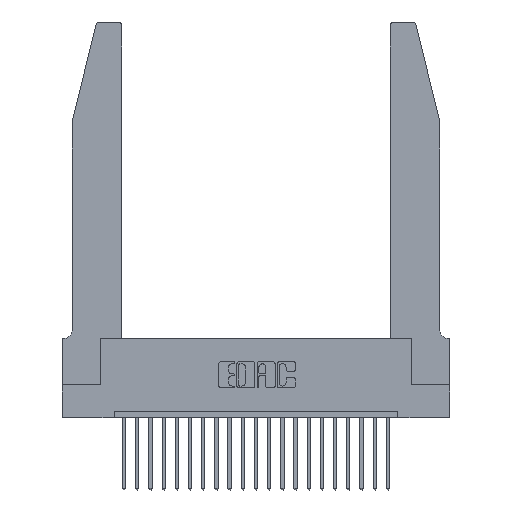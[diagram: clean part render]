
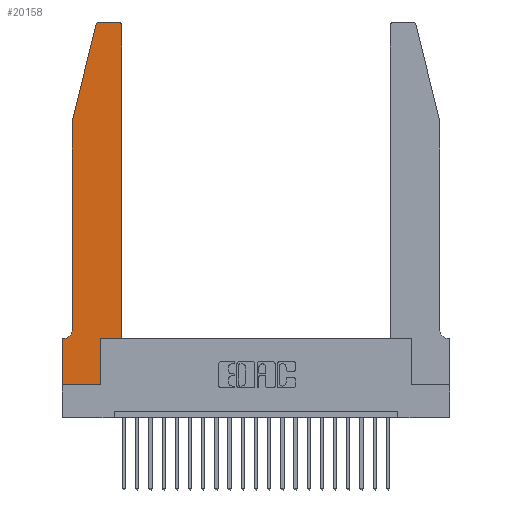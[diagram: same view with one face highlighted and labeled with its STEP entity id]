
A CAD part, top view. The second image highlights one B-rep face of the part: STEP entity #20158.
In plain terms, the highlighted planar face has unit normal (0, 0, 1).
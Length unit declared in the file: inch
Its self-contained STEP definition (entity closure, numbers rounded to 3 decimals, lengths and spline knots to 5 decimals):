
#213 = VECTOR ( 'NONE', #15141, 39.37008 ) ;
#863 = CARTESIAN_POINT ( 'NONE',  ( 0.284, 2.72, 0.37 ) ) ;
#1132 = VECTOR ( 'NONE', #19021, 39.37008 ) ;
#1292 = VECTOR ( 'NONE', #7673, 39.37008 ) ;
#1314 = CARTESIAN_POINT ( 'NONE',  ( 0.4505, 2.72, 0.37 ) ) ;
#1641 = ORIENTED_EDGE ( 'NONE', *, *, #21654, .T. ) ;
#2424 = VERTEX_POINT ( 'NONE', #9482 ) ;
#2487 = EDGE_CURVE ( 'NONE', #17698, #15818, #4544, .T. ) ;
#2491 = VERTEX_POINT ( 'NONE', #2927 ) ;
#2631 = CARTESIAN_POINT ( 'NONE',  ( 0.2605, 2.75, 0.37 ) ) ;
#2733 = AXIS2_PLACEMENT_3D ( 'NONE', #9581, #9657, #7520 ) ;
#2805 = EDGE_CURVE ( 'NONE', #15322, #13369, #13074, .T. ) ;
#2927 = CARTESIAN_POINT ( 'NONE',  ( 0.284, 2.75, 0.37 ) ) ;
#3607 = VECTOR ( 'NONE', #6614, 39.37008 ) ;
#3622 = EDGE_CURVE ( 'NONE', #21096, #16097, #10498, .T. ) ;
#3660 = DIRECTION ( 'NONE',  ( -0.239, -0.971, 0. ) ) ;
#3994 = EDGE_CURVE ( 'NONE', #9975, #22409, #5605, .T. ) ;
#4544 = LINE ( 'NONE', #19056, #6535 ) ;
#5155 = EDGE_CURVE ( 'NONE', #13369, #9975, #8724, .T. ) ;
#5460 = EDGE_CURVE ( 'NONE', #15818, #21096, #10680, .T. ) ;
#5528 = AXIS2_PLACEMENT_3D ( 'NONE', #863, #13330, #11585 ) ;
#5605 = CIRCLE ( 'NONE', #13168, 0.03 ) ;
#6391 = ORIENTED_EDGE ( 'NONE', *, *, #12423, .T. ) ;
#6535 = VECTOR ( 'NONE', #19134, 39.37008 ) ;
#6614 = DIRECTION ( 'NONE',  ( 0., 1., 0. ) ) ;
#6942 = CARTESIAN_POINT ( 'NONE',  ( 0.2865, 0., 0.37 ) ) ;
#7028 = CARTESIAN_POINT ( 'NONE',  ( 0.4505, 0.35, 0.37 ) ) ;
#7123 = VERTEX_POINT ( 'NONE', #14315 ) ;
#7237 = LINE ( 'NONE', #2631, #1292 ) ;
#7520 = DIRECTION ( 'NONE',  ( 1., 0., 0. ) ) ;
#7673 = DIRECTION ( 'NONE',  ( -1., 0., 0. ) ) ;
#7934 = CIRCLE ( 'NONE', #18962, 0.07 ) ;
#8153 = EDGE_CURVE ( 'NONE', #7123, #17698, #7934, .T. ) ;
#8240 = CARTESIAN_POINT ( 'NONE',  ( 0., 0., 0.37 ) ) ;
#8246 = ORIENTED_EDGE ( 'NONE', *, *, #3622, .T. ) ;
#8338 = CARTESIAN_POINT ( 'NONE',  ( 0.4505, 0.35, 0.37 ) ) ;
#8724 = LINE ( 'NONE', #21143, #3607 ) ;
#9340 = DIRECTION ( 'NONE',  ( 0., 0., -1. ) ) ;
#9482 = CARTESIAN_POINT ( 'NONE',  ( 0.25487, 2.72718, 0.37 ) ) ;
#9508 = ORIENTED_EDGE ( 'NONE', *, *, #3994, .T. ) ;
#9581 = CARTESIAN_POINT ( 'NONE',  ( 0., 0.35, 0.37 ) ) ;
#9646 = DIRECTION ( 'NONE',  ( -1., 0., 0. ) ) ;
#9657 = DIRECTION ( 'NONE',  ( 0., 0., 1. ) ) ;
#9975 = VERTEX_POINT ( 'NONE', #1314 ) ;
#10147 = LINE ( 'NONE', #17157, #213 ) ;
#10498 = LINE ( 'NONE', #16971, #1132 ) ;
#10680 = LINE ( 'NONE', #22057, #14885 ) ;
#10741 = VERTEX_POINT ( 'NONE', #18191 ) ;
#10784 = CARTESIAN_POINT ( 'NONE',  ( 0.0755, 2., 0.37 ) ) ;
#11191 = CARTESIAN_POINT ( 'NONE',  ( 0.0055, 0.42, 0.37 ) ) ;
#11566 = ORIENTED_EDGE ( 'NONE', *, *, #2487, .T. ) ;
#11585 = DIRECTION ( 'NONE',  ( 1., 0., 0. ) ) ;
#11810 = CARTESIAN_POINT ( 'NONE',  ( 0., 0.35, 0.37 ) ) ;
#12199 = ORIENTED_EDGE ( 'NONE', *, *, #5460, .T. ) ;
#12423 = EDGE_CURVE ( 'NONE', #2424, #10741, #23289, .T. ) ;
#12503 = DIRECTION ( 'NONE',  ( 1., 0., 0. ) ) ;
#12943 = DIRECTION ( 'NONE',  ( 1., 0., 0. ) ) ;
#12972 = LINE ( 'NONE', #19610, #14895 ) ;
#13074 = LINE ( 'NONE', #7028, #20637 ) ;
#13104 = PLANE ( 'NONE',  #2733 ) ;
#13168 = AXIS2_PLACEMENT_3D ( 'NONE', #14573, #14716, #12943 ) ;
#13330 = DIRECTION ( 'NONE',  ( 0., 0., 1. ) ) ;
#13369 = VERTEX_POINT ( 'NONE', #8338 ) ;
#13471 = CARTESIAN_POINT ( 'NONE',  ( 0.2865, 0.35, 0.37 ) ) ;
#14315 = CARTESIAN_POINT ( 'NONE',  ( 0.0755, 0.42, 0.37 ) ) ;
#14573 = CARTESIAN_POINT ( 'NONE',  ( 0.4205, 2.72, 0.37 ) ) ;
#14648 = ORIENTED_EDGE ( 'NONE', *, *, #5155, .T. ) ;
#14716 = DIRECTION ( 'NONE',  ( 0., 0., 1. ) ) ;
#14883 = DIRECTION ( 'NONE',  ( 0., -1., 0. ) ) ;
#14885 = VECTOR ( 'NONE', #14883, 39.37008 ) ;
#14895 = VECTOR ( 'NONE', #21388, 39.37008 ) ;
#15141 = DIRECTION ( 'NONE',  ( 0., 1., 0. ) ) ;
#15322 = VERTEX_POINT ( 'NONE', #13471 ) ;
#15744 = ORIENTED_EDGE ( 'NONE', *, *, #15996, .T. ) ;
#15818 = VERTEX_POINT ( 'NONE', #11810 ) ;
#15996 = EDGE_CURVE ( 'NONE', #22409, #2491, #7237, .T. ) ;
#16097 = VERTEX_POINT ( 'NONE', #6942 ) ;
#16695 = ORIENTED_EDGE ( 'NONE', *, *, #8153, .T. ) ;
#16971 = CARTESIAN_POINT ( 'NONE',  ( 0., 0., 0.37 ) ) ;
#17157 = CARTESIAN_POINT ( 'NONE',  ( 0.2865, 0.35, 0.37 ) ) ;
#17166 = ORIENTED_EDGE ( 'NONE', *, *, #2805, .T. ) ;
#17698 = VERTEX_POINT ( 'NONE', #22818 ) ;
#18191 = CARTESIAN_POINT ( 'NONE',  ( 0.0755, 2., 0.37 ) ) ;
#18418 = EDGE_CURVE ( 'NONE', #2491, #2424, #21782, .T. ) ;
#18620 = ORIENTED_EDGE ( 'NONE', *, *, #23187, .T. ) ;
#18962 = AXIS2_PLACEMENT_3D ( 'NONE', #11191, #9340, #9646 ) ;
#19021 = DIRECTION ( 'NONE',  ( 1., 0., 0. ) ) ;
#19056 = CARTESIAN_POINT ( 'NONE',  ( 0.0755, 0.35, 0.37 ) ) ;
#19134 = DIRECTION ( 'NONE',  ( -1., 0., 0. ) ) ;
#19610 = CARTESIAN_POINT ( 'NONE',  ( 0.0755, 2., 0.37 ) ) ;
#19623 = VECTOR ( 'NONE', #3660, 39.37008 ) ;
#20158 = ADVANCED_FACE ( 'NONE', ( #21723 ), #13104, .T. ) ;
#20637 = VECTOR ( 'NONE', #12503, 39.37008 ) ;
#21096 = VERTEX_POINT ( 'NONE', #8240 ) ;
#21143 = CARTESIAN_POINT ( 'NONE',  ( 0.4505, 0.35, 0.37 ) ) ;
#21388 = DIRECTION ( 'NONE',  ( 0., -1., 0. ) ) ;
#21654 = EDGE_CURVE ( 'NONE', #16097, #15322, #10147, .T. ) ;
#21723 = FACE_OUTER_BOUND ( 'NONE', #23404, .T. ) ;
#21782 = CIRCLE ( 'NONE', #5528, 0.03 ) ;
#22035 = ORIENTED_EDGE ( 'NONE', *, *, #18418, .T. ) ;
#22057 = CARTESIAN_POINT ( 'NONE',  ( 0., 0., 0.37 ) ) ;
#22376 = CARTESIAN_POINT ( 'NONE',  ( 0.4205, 2.75, 0.37 ) ) ;
#22409 = VERTEX_POINT ( 'NONE', #22376 ) ;
#22818 = CARTESIAN_POINT ( 'NONE',  ( 0.0055, 0.35, 0.37 ) ) ;
#23187 = EDGE_CURVE ( 'NONE', #10741, #7123, #12972, .T. ) ;
#23289 = LINE ( 'NONE', #10784, #19623 ) ;
#23404 = EDGE_LOOP ( 'NONE', ( #15744, #22035, #6391, #18620, #16695, #11566, #12199, #8246, #1641, #17166, #14648, #9508 ) ) ;
